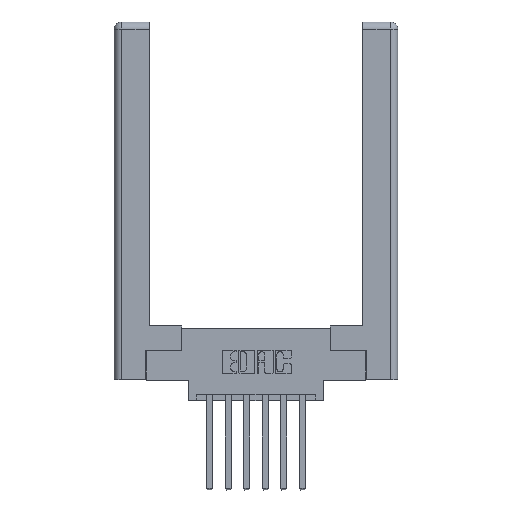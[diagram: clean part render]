
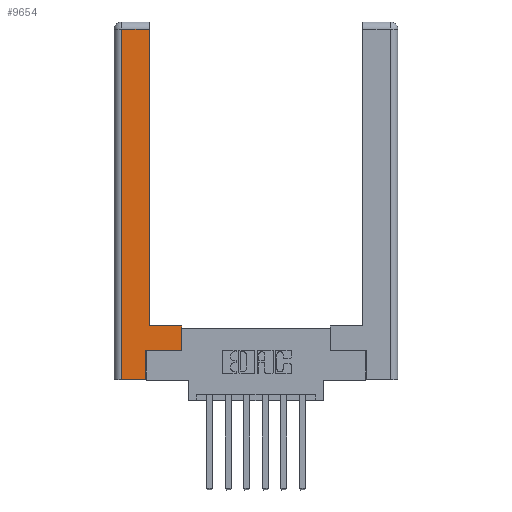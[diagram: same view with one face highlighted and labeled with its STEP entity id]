
A CAD part, top view. The second image highlights one B-rep face of the part: STEP entity #9654.
In plain terms, the highlighted planar face has unit normal (0, 0, 1).
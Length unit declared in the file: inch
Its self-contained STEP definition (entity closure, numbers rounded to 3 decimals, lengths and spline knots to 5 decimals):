
#245 = EDGE_CURVE ( 'NONE', #7951, #6555, #5837, .T. ) ;
#542 = DIRECTION ( 'NONE',  ( 0., -1., 0. ) ) ;
#768 = ORIENTED_EDGE ( 'NONE', *, *, #11555, .T. ) ;
#1112 = EDGE_CURVE ( 'NONE', #3387, #5564, #5815, .T. ) ;
#1218 = EDGE_CURVE ( 'NONE', #7911, #3323, #8092, .T. ) ;
#1334 = CARTESIAN_POINT ( 'NONE',  ( 0.0615, 0., 0. ) ) ;
#1403 = AXIS2_PLACEMENT_3D ( 'NONE', #2520, #1630, #11651 ) ;
#1630 = DIRECTION ( 'NONE',  ( 0., 0., -1. ) ) ;
#1826 = LINE ( 'NONE', #8495, #9609 ) ;
#2225 = VECTOR ( 'NONE', #10515, 39.37008 ) ;
#2355 = CARTESIAN_POINT ( 'NONE',  ( 0.565, 0.245, 0. ) ) ;
#2405 = PLANE ( 'NONE',  #1403 ) ;
#2453 = CARTESIAN_POINT ( 'NONE',  ( 0.0615, 0., 0. ) ) ;
#2520 = CARTESIAN_POINT ( 'NONE',  ( 0., 0., 0. ) ) ;
#2973 = DIRECTION ( 'NONE',  ( -1., 0., 0. ) ) ;
#3323 = VERTEX_POINT ( 'NONE', #2355 ) ;
#3387 = VERTEX_POINT ( 'NONE', #1334 ) ;
#3390 = CARTESIAN_POINT ( 'NONE',  ( 0.0615, 2.94, 0. ) ) ;
#3455 = ORIENTED_EDGE ( 'NONE', *, *, #4713, .T. ) ;
#3913 = CARTESIAN_POINT ( 'NONE',  ( 0.295, 0.45, 0. ) ) ;
#3940 = ORIENTED_EDGE ( 'NONE', *, *, #245, .T. ) ;
#3966 = LINE ( 'NONE', #5084, #2225 ) ;
#4066 = ORIENTED_EDGE ( 'NONE', *, *, #1218, .T. ) ;
#4123 = VECTOR ( 'NONE', #4927, 39.37008 ) ;
#4607 = EDGE_CURVE ( 'NONE', #5612, #8528, #1826, .T. ) ;
#4713 = EDGE_CURVE ( 'NONE', #5564, #7911, #9767, .T. ) ;
#4927 = DIRECTION ( 'NONE',  ( 0., 1., 0. ) ) ;
#4997 = CARTESIAN_POINT ( 'NONE',  ( 0.295, 3., 0. ) ) ;
#5084 = CARTESIAN_POINT ( 'NONE',  ( 0.565, 0.45, 0. ) ) ;
#5250 = LINE ( 'NONE', #2453, #11412 ) ;
#5368 = VECTOR ( 'NONE', #9896, 39.37008 ) ;
#5564 = VERTEX_POINT ( 'NONE', #9542 ) ;
#5608 = EDGE_CURVE ( 'NONE', #8528, #7951, #7454, .T. ) ;
#5612 = VERTEX_POINT ( 'NONE', #5854 ) ;
#5815 = LINE ( 'NONE', #9079, #10281 ) ;
#5837 = LINE ( 'NONE', #3390, #6709 ) ;
#5854 = CARTESIAN_POINT ( 'NONE',  ( 0.565, 0.45, 0. ) ) ;
#6347 = CARTESIAN_POINT ( 'NONE',  ( 0.565, 0.245, 0. ) ) ;
#6555 = VERTEX_POINT ( 'NONE', #10059 ) ;
#6709 = VECTOR ( 'NONE', #10763, 39.37008 ) ;
#7022 = CARTESIAN_POINT ( 'NONE',  ( 0.265, 0.245, 0. ) ) ;
#7298 = EDGE_LOOP ( 'NONE', ( #7712, #3940, #768, #7768, #3455, #4066, #10388, #11450 ) ) ;
#7334 = VECTOR ( 'NONE', #11578, 39.37008 ) ;
#7454 = LINE ( 'NONE', #4997, #4123 ) ;
#7468 = CARTESIAN_POINT ( 'NONE',  ( 0.265, 0.245, 0. ) ) ;
#7712 = ORIENTED_EDGE ( 'NONE', *, *, #5608, .T. ) ;
#7768 = ORIENTED_EDGE ( 'NONE', *, *, #1112, .T. ) ;
#7911 = VERTEX_POINT ( 'NONE', #7468 ) ;
#7951 = VERTEX_POINT ( 'NONE', #10243 ) ;
#8092 = LINE ( 'NONE', #6347, #5368 ) ;
#8495 = CARTESIAN_POINT ( 'NONE',  ( 0.295, 0.45, 0. ) ) ;
#8528 = VERTEX_POINT ( 'NONE', #3913 ) ;
#9002 = DIRECTION ( 'NONE',  ( 1., 0., 0. ) ) ;
#9079 = CARTESIAN_POINT ( 'NONE',  ( 0.265, 0., 0. ) ) ;
#9542 = CARTESIAN_POINT ( 'NONE',  ( 0.265, 0., 0. ) ) ;
#9609 = VECTOR ( 'NONE', #2973, 39.37008 ) ;
#9654 = ADVANCED_FACE ( 'NONE', ( #10349 ), #2405, .F. ) ;
#9767 = LINE ( 'NONE', #7022, #7334 ) ;
#9896 = DIRECTION ( 'NONE',  ( 1., 0., 0. ) ) ;
#10059 = CARTESIAN_POINT ( 'NONE',  ( 0.0615, 2.94, 0. ) ) ;
#10243 = CARTESIAN_POINT ( 'NONE',  ( 0.295, 2.94, 0. ) ) ;
#10281 = VECTOR ( 'NONE', #9002, 39.37008 ) ;
#10349 = FACE_OUTER_BOUND ( 'NONE', #7298, .T. ) ;
#10388 = ORIENTED_EDGE ( 'NONE', *, *, #11021, .T. ) ;
#10515 = DIRECTION ( 'NONE',  ( 0., 1., 0. ) ) ;
#10763 = DIRECTION ( 'NONE',  ( -1., 0., 0. ) ) ;
#11021 = EDGE_CURVE ( 'NONE', #3323, #5612, #3966, .T. ) ;
#11412 = VECTOR ( 'NONE', #542, 39.37008 ) ;
#11450 = ORIENTED_EDGE ( 'NONE', *, *, #4607, .T. ) ;
#11555 = EDGE_CURVE ( 'NONE', #6555, #3387, #5250, .T. ) ;
#11578 = DIRECTION ( 'NONE',  ( 0., 1., 0. ) ) ;
#11651 = DIRECTION ( 'NONE',  ( -1., 0., 0. ) ) ;
